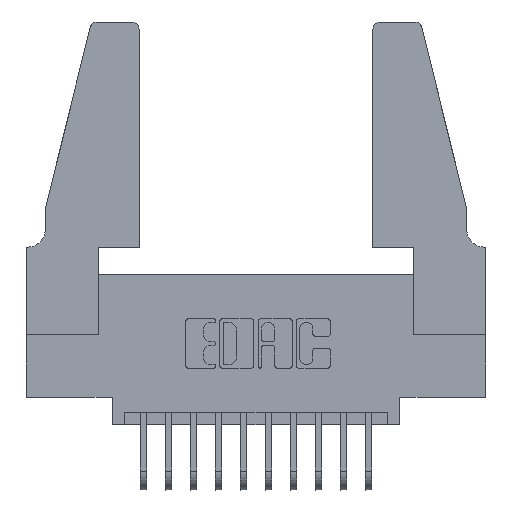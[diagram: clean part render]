
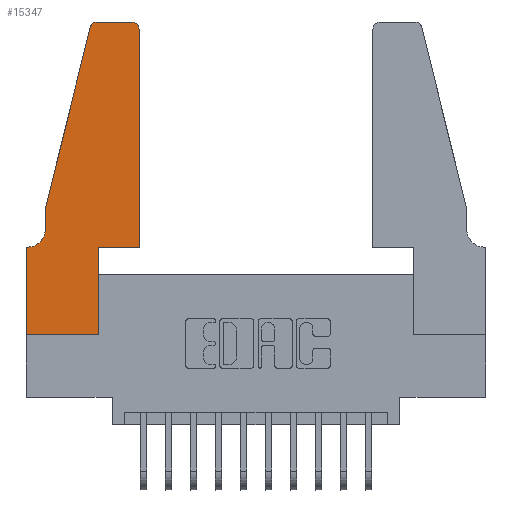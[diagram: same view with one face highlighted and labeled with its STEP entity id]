
A CAD part, top view. The second image highlights one B-rep face of the part: STEP entity #15347.
In plain terms, the highlighted planar face has unit normal (0, 0, 1).
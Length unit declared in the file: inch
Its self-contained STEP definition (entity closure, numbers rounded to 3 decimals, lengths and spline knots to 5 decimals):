
#201 = CARTESIAN_POINT ( 'NONE',  ( 0., 0.35, 0.37 ) ) ;
#221 = DIRECTION ( 'NONE',  ( 0., -1., 0. ) ) ;
#228 = CARTESIAN_POINT ( 'NONE',  ( 0.4505, 0.35, 0.37 ) ) ;
#608 = VERTEX_POINT ( 'NONE', #14344 ) ;
#1029 = AXIS2_PLACEMENT_3D ( 'NONE', #6308, #8801, #1389 ) ;
#1141 = EDGE_CURVE ( 'NONE', #10293, #11214, #9005, .T. ) ;
#1188 = ORIENTED_EDGE ( 'NONE', *, *, #1141, .T. ) ;
#1198 = ORIENTED_EDGE ( 'NONE', *, *, #2166, .T. ) ;
#1389 = DIRECTION ( 'NONE',  ( 1., 0., 0. ) ) ;
#1731 = DIRECTION ( 'NONE',  ( 0., -1., 0. ) ) ;
#1733 = VECTOR ( 'NONE', #8838, 39.37008 ) ;
#1869 = ORIENTED_EDGE ( 'NONE', *, *, #11908, .T. ) ;
#2007 = LINE ( 'NONE', #7727, #4914 ) ;
#2023 = ORIENTED_EDGE ( 'NONE', *, *, #2307, .T. ) ;
#2041 = CARTESIAN_POINT ( 'NONE',  ( 0.0055, 0.42, 0.37 ) ) ;
#2166 = EDGE_CURVE ( 'NONE', #3543, #3445, #2007, .T. ) ;
#2275 = AXIS2_PLACEMENT_3D ( 'NONE', #4894, #13545, #6135 ) ;
#2307 = EDGE_CURVE ( 'NONE', #11214, #3543, #8772, .T. ) ;
#2562 = ORIENTED_EDGE ( 'NONE', *, *, #5735, .T. ) ;
#2819 = ORIENTED_EDGE ( 'NONE', *, *, #4613, .T. ) ;
#3199 = VERTEX_POINT ( 'NONE', #14673 ) ;
#3275 = LINE ( 'NONE', #4222, #15662 ) ;
#3287 = DIRECTION ( 'NONE',  ( -1., 0., 0. ) ) ;
#3337 = ORIENTED_EDGE ( 'NONE', *, *, #12796, .T. ) ;
#3400 = VECTOR ( 'NONE', #221, 39.37008 ) ;
#3441 = EDGE_LOOP ( 'NONE', ( #15238, #7498, #5031, #8495, #3668, #2562, #3337, #1188, #2023, #1198, #2819, #1869 ) ) ;
#3445 = VERTEX_POINT ( 'NONE', #228 ) ;
#3543 = VERTEX_POINT ( 'NONE', #14072 ) ;
#3668 = ORIENTED_EDGE ( 'NONE', *, *, #5814, .T. ) ;
#3967 = EDGE_CURVE ( 'NONE', #608, #8809, #14731, .T. ) ;
#4222 = CARTESIAN_POINT ( 'NONE',  ( 0., 0., 0.37 ) ) ;
#4313 = DIRECTION ( 'NONE',  ( 0., 1., 0. ) ) ;
#4613 = EDGE_CURVE ( 'NONE', #3445, #6407, #8315, .T. ) ;
#4705 = AXIS2_PLACEMENT_3D ( 'NONE', #5271, #13895, #6482 ) ;
#4798 = CARTESIAN_POINT ( 'NONE',  ( 0., 0., 0.37 ) ) ;
#4850 = VECTOR ( 'NONE', #7676, 39.37008 ) ;
#4894 = CARTESIAN_POINT ( 'NONE',  ( 0.4205, 1.22, 0.37 ) ) ;
#4899 = AXIS2_PLACEMENT_3D ( 'NONE', #2041, #10691, #3287 ) ;
#4914 = VECTOR ( 'NONE', #10157, 39.37008 ) ;
#5031 = ORIENTED_EDGE ( 'NONE', *, *, #12939, .T. ) ;
#5271 = CARTESIAN_POINT ( 'NONE',  ( 0.284, 1.22, 0.37 ) ) ;
#5518 = EDGE_CURVE ( 'NONE', #6885, #6476, #9583, .T. ) ;
#5706 = CARTESIAN_POINT ( 'NONE',  ( 0.4505, 1.22, 0.37 ) ) ;
#5716 = CIRCLE ( 'NONE', #4899, 0.07 ) ;
#5731 = DIRECTION ( 'NONE',  ( -0.239, -0.971, 0. ) ) ;
#5735 = EDGE_CURVE ( 'NONE', #3199, #6143, #12685, .T. ) ;
#5814 = EDGE_CURVE ( 'NONE', #6476, #3199, #5716, .T. ) ;
#6135 = DIRECTION ( 'NONE',  ( 1., 0., 0. ) ) ;
#6143 = VERTEX_POINT ( 'NONE', #201 ) ;
#6308 = CARTESIAN_POINT ( 'NONE',  ( 0., 0.35, 0.37 ) ) ;
#6407 = VERTEX_POINT ( 'NONE', #5706 ) ;
#6431 = CARTESIAN_POINT ( 'NONE',  ( 0.2605, 1.25, 0.37 ) ) ;
#6476 = VERTEX_POINT ( 'NONE', #15711 ) ;
#6482 = DIRECTION ( 'NONE',  ( 1., 0., 0. ) ) ;
#6550 = CARTESIAN_POINT ( 'NONE',  ( 0.0755, 0.5, 0.37 ) ) ;
#6793 = CARTESIAN_POINT ( 'NONE',  ( 0.284, 1.25, 0.37 ) ) ;
#6885 = VERTEX_POINT ( 'NONE', #6550 ) ;
#7466 = EDGE_CURVE ( 'NONE', #8809, #15090, #14018, .T. ) ;
#7498 = ORIENTED_EDGE ( 'NONE', *, *, #7466, .T. ) ;
#7676 = DIRECTION ( 'NONE',  ( -1., 0., 0. ) ) ;
#7680 = CARTESIAN_POINT ( 'NONE',  ( 0.0755, 0.5, 0.37 ) ) ;
#7727 = CARTESIAN_POINT ( 'NONE',  ( 0.4505, 0.35, 0.37 ) ) ;
#7865 = FACE_OUTER_BOUND ( 'NONE', #3441, .T. ) ;
#8045 = DIRECTION ( 'NONE',  ( 1., 0., 0. ) ) ;
#8135 = CARTESIAN_POINT ( 'NONE',  ( 0., 0., 0.37 ) ) ;
#8315 = LINE ( 'NONE', #10086, #1733 ) ;
#8495 = ORIENTED_EDGE ( 'NONE', *, *, #5518, .T. ) ;
#8772 = LINE ( 'NONE', #11710, #9145 ) ;
#8801 = DIRECTION ( 'NONE',  ( 0., 0., 1. ) ) ;
#8809 = VERTEX_POINT ( 'NONE', #6793 ) ;
#8838 = DIRECTION ( 'NONE',  ( 0., 1., 0. ) ) ;
#9005 = LINE ( 'NONE', #8135, #9770 ) ;
#9145 = VECTOR ( 'NONE', #4313, 39.37008 ) ;
#9372 = VECTOR ( 'NONE', #13012, 39.37008 ) ;
#9583 = LINE ( 'NONE', #7680, #3400 ) ;
#9770 = VECTOR ( 'NONE', #8045, 39.37008 ) ;
#10041 = VECTOR ( 'NONE', #5731, 39.37008 ) ;
#10086 = CARTESIAN_POINT ( 'NONE',  ( 0.4505, 0.35, 0.37 ) ) ;
#10157 = DIRECTION ( 'NONE',  ( 1., 0., 0. ) ) ;
#10293 = VERTEX_POINT ( 'NONE', #4798 ) ;
#10431 = LINE ( 'NONE', #11881, #10041 ) ;
#10691 = DIRECTION ( 'NONE',  ( 0., 0., -1. ) ) ;
#11214 = VERTEX_POINT ( 'NONE', #14491 ) ;
#11710 = CARTESIAN_POINT ( 'NONE',  ( 0.2865, 0.35, 0.37 ) ) ;
#11881 = CARTESIAN_POINT ( 'NONE',  ( 0.0755, 0.5, 0.37 ) ) ;
#11908 = EDGE_CURVE ( 'NONE', #6407, #608, #14538, .T. ) ;
#11997 = CARTESIAN_POINT ( 'NONE',  ( 0.25487, 1.22718, 0.37 ) ) ;
#12483 = PLANE ( 'NONE',  #1029 ) ;
#12685 = LINE ( 'NONE', #15463, #9372 ) ;
#12796 = EDGE_CURVE ( 'NONE', #6143, #10293, #3275, .T. ) ;
#12939 = EDGE_CURVE ( 'NONE', #15090, #6885, #10431, .T. ) ;
#13012 = DIRECTION ( 'NONE',  ( -1., 0., 0. ) ) ;
#13545 = DIRECTION ( 'NONE',  ( 0., 0., 1. ) ) ;
#13895 = DIRECTION ( 'NONE',  ( 0., 0., 1. ) ) ;
#14018 = CIRCLE ( 'NONE', #4705, 0.03 ) ;
#14072 = CARTESIAN_POINT ( 'NONE',  ( 0.2865, 0.35, 0.37 ) ) ;
#14344 = CARTESIAN_POINT ( 'NONE',  ( 0.4205, 1.25, 0.37 ) ) ;
#14491 = CARTESIAN_POINT ( 'NONE',  ( 0.2865, 0., 0.37 ) ) ;
#14538 = CIRCLE ( 'NONE', #2275, 0.03 ) ;
#14673 = CARTESIAN_POINT ( 'NONE',  ( 0.0055, 0.35, 0.37 ) ) ;
#14731 = LINE ( 'NONE', #6431, #4850 ) ;
#15090 = VERTEX_POINT ( 'NONE', #11997 ) ;
#15238 = ORIENTED_EDGE ( 'NONE', *, *, #3967, .T. ) ;
#15347 = ADVANCED_FACE ( 'NONE', ( #7865 ), #12483, .T. ) ;
#15463 = CARTESIAN_POINT ( 'NONE',  ( 0.0755, 0.35, 0.37 ) ) ;
#15662 = VECTOR ( 'NONE', #1731, 39.37008 ) ;
#15711 = CARTESIAN_POINT ( 'NONE',  ( 0.0755, 0.42, 0.37 ) ) ;
